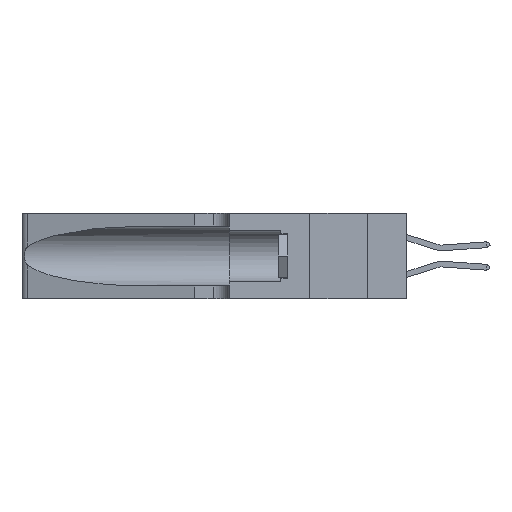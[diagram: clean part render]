
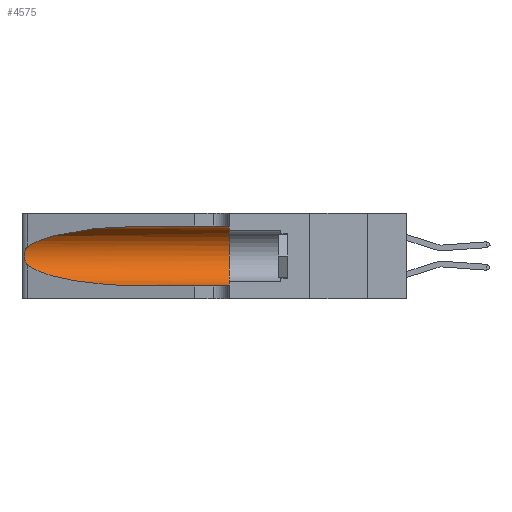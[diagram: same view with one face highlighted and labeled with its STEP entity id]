
A CAD part, left-side view. The second image highlights one B-rep face of the part: STEP entity #4575.
In plain terms, the highlighted cylindrical face has radius 3.308 mm (diameter 6.617 mm), a partial arc.
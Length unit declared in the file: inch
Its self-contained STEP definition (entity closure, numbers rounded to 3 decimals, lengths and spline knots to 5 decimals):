
#116 = CARTESIAN_POINT ( 'NONE',  ( 0.1305, 0.35, 0.05475 ) ) ;
#204 = CARTESIAN_POINT ( 'NONE',  ( 0.25854, 1.2359, 0.20912 ) ) ;
#743 = VERTEX_POINT ( 'NONE', #1763 ) ;
#820 = CARTESIAN_POINT ( 'NONE',  ( 0.1305, 0.35, 0.31525 ) ) ;
#1292 = DIRECTION ( 'NONE',  ( 0., 1., 0. ) ) ;
#1763 = CARTESIAN_POINT ( 'NONE',  ( 0.25487, 1.22718, 0.14631 ) ) ;
#1822 = ORIENTED_EDGE ( 'NONE', *, *, #18909, .T. ) ;
#2095 = EDGE_CURVE ( 'NONE', #21212, #743, #15231, .T. ) ;
#3224 = EDGE_CURVE ( 'NONE', #14481, #21212, #11499, .T. ) ;
#3619 = CARTESIAN_POINT ( 'NONE',  ( 0.1305, 1.61858, 0.05475 ) ) ;
#3789 = CARTESIAN_POINT ( 'NONE',  ( 0.25555, 1.22994, 0.2215 ) ) ;
#3817 = CARTESIAN_POINT ( 'NONE',  ( 0.26018, 1.23835, 0.19895 ) ) ;
#3951 = CARTESIAN_POINT ( 'NONE',  ( 0.25856, 1.23593, 0.16098 ) ) ;
#4509 = CARTESIAN_POINT ( 'NONE',  ( 0.25789, 1.23486, 0.15765 ) ) ;
#4575 = ADVANCED_FACE ( 'NONE', ( #9267 ), #12246, .F. ) ;
#5392 = ORIENTED_EDGE ( 'NONE', *, *, #2095, .T. ) ;
#6337 = ORIENTED_EDGE ( 'NONE', *, *, #8643, .F. ) ;
#6398 = CARTESIAN_POINT ( 'NONE',  ( 0.1305, 0.72297, 0.05475 ) ) ;
#6425 = CARTESIAN_POINT ( 'NONE',  ( 0.25487, 1.22718, 0.22369 ) ) ;
#7022 = VERTEX_POINT ( 'NONE', #20162 ) ;
#7311 = EDGE_CURVE ( 'NONE', #743, #7022, #11792, .T. ) ;
#7464 = CARTESIAN_POINT ( 'NONE',  ( 0.1305, 1.61858, 0.31525 ) ) ;
#7591 = AXIS2_PLACEMENT_3D ( 'NONE', #8154, #1292, #13288 ) ;
#8154 = CARTESIAN_POINT ( 'NONE',  ( 0.1305, 0.35, 0.185 ) ) ;
#8545 = LINE ( 'NONE', #7464, #14473 ) ;
#8599 = EDGE_CURVE ( 'NONE', #14481, #14211, #8545, .T. ) ;
#8643 = EDGE_CURVE ( 'NONE', #14211, #12919, #10958, .T. ) ;
#8984 = CARTESIAN_POINT ( 'NONE',  ( 0.25487, 1.22718, 0.14631 ) ) ;
#9267 = FACE_OUTER_BOUND ( 'NONE', #21830, .T. ) ;
#10089 = CARTESIAN_POINT ( 'NONE',  ( 0.1305, 1.61858, 0.185 ) ) ;
#10958 = CIRCLE ( 'NONE', #7591, 0.13025 ) ;
#11499 =( BOUNDED_CURVE ( )  B_SPLINE_CURVE ( 3, ( #16228, #17680, #14275, #12471 ),
 .UNSPECIFIED., .F., .T. ) 
 B_SPLINE_CURVE_WITH_KNOTS ( ( 4, 4 ),
 ( 1.5708, 2.84003 ),
 .UNSPECIFIED. ) 
 CURVE ( )  GEOMETRIC_REPRESENTATION_ITEM ( )  RATIONAL_B_SPLINE_CURVE ( ( 1., 0.87, 0.87, 1. ) ) 
 REPRESENTATION_ITEM ( '' )  );
#11741 = CARTESIAN_POINT ( 'NONE',  ( 0.18966, 0.96281, 0.05475 ) ) ;
#11792 =( BOUNDED_CURVE ( )  B_SPLINE_CURVE ( 3, ( #8984, #15050, #11741, #6398 ),
 .UNSPECIFIED., .F., .T. ) 
 B_SPLINE_CURVE_WITH_KNOTS ( ( 4, 4 ),
 ( 3.44316, 4.71239 ),
 .UNSPECIFIED. ) 
 CURVE ( )  GEOMETRIC_REPRESENTATION_ITEM ( )  RATIONAL_B_SPLINE_CURVE ( ( 1., 0.87, 0.87, 1. ) ) 
 REPRESENTATION_ITEM ( '' )  );
#12246 = CYLINDRICAL_SURFACE ( 'NONE', #14768, 0.13025 ) ;
#12471 = CARTESIAN_POINT ( 'NONE',  ( 0.25487, 1.22718, 0.22369 ) ) ;
#12919 = VERTEX_POINT ( 'NONE', #116 ) ;
#13288 = DIRECTION ( 'NONE',  ( 0., 0., 1. ) ) ;
#13420 = ORIENTED_EDGE ( 'NONE', *, *, #8599, .F. ) ;
#13934 = CARTESIAN_POINT ( 'NONE',  ( 0.25639, 1.23184, 0.21858 ) ) ;
#14068 = CARTESIAN_POINT ( 'NONE',  ( 0.25787, 1.23484, 0.2124 ) ) ;
#14211 = VERTEX_POINT ( 'NONE', #820 ) ;
#14275 = CARTESIAN_POINT ( 'NONE',  ( 0.2373, 1.15595, 0.28018 ) ) ;
#14473 = VECTOR ( 'NONE', #21308, 39.37008 ) ;
#14481 = VERTEX_POINT ( 'NONE', #17709 ) ;
#14768 = AXIS2_PLACEMENT_3D ( 'NONE', #10089, #16945, #22263 ) ;
#15050 = CARTESIAN_POINT ( 'NONE',  ( 0.2373, 1.15595, 0.08982 ) ) ;
#15213 = CARTESIAN_POINT ( 'NONE',  ( 0.25555, 1.22993, 0.14849 ) ) ;
#15231 = B_SPLINE_CURVE_WITH_KNOTS ( 'NONE', 3,
 ( #15700, #3789, #13934, #14068, #204, #3817, #15857, #17625, #19977, #3951, #4509, #15936, #15213, #16944 ),
 .UNSPECIFIED., .F., .F.,
 ( 4, 2, 2, 2, 2, 2, 4 ),
 ( 0., 0.00027, 0.00053, 0.00107, 0.0016, 0.00187, 0.00214 ),
 .UNSPECIFIED. ) ;
#15674 = ORIENTED_EDGE ( 'NONE', *, *, #7311, .T. ) ;
#15700 = CARTESIAN_POINT ( 'NONE',  ( 0.25487, 1.22718, 0.22369 ) ) ;
#15857 = CARTESIAN_POINT ( 'NONE',  ( 0.26075, 1.23896, 0.19203 ) ) ;
#15867 = VECTOR ( 'NONE', #20923, 39.37008 ) ;
#15936 = CARTESIAN_POINT ( 'NONE',  ( 0.25639, 1.23186, 0.15144 ) ) ;
#16228 = CARTESIAN_POINT ( 'NONE',  ( 0.1305, 0.72297, 0.31525 ) ) ;
#16944 = CARTESIAN_POINT ( 'NONE',  ( 0.25487, 1.22718, 0.14631 ) ) ;
#16945 = DIRECTION ( 'NONE',  ( 0., -1., 0. ) ) ;
#17625 = CARTESIAN_POINT ( 'NONE',  ( 0.26075, 1.23896, 0.178 ) ) ;
#17680 = CARTESIAN_POINT ( 'NONE',  ( 0.18966, 0.96281, 0.31525 ) ) ;
#17709 = CARTESIAN_POINT ( 'NONE',  ( 0.1305, 0.72297, 0.31525 ) ) ;
#18909 = EDGE_CURVE ( 'NONE', #7022, #12919, #20244, .T. ) ;
#19521 = ORIENTED_EDGE ( 'NONE', *, *, #3224, .T. ) ;
#19977 = CARTESIAN_POINT ( 'NONE',  ( 0.26017, 1.23833, 0.17102 ) ) ;
#20162 = CARTESIAN_POINT ( 'NONE',  ( 0.1305, 0.72297, 0.05475 ) ) ;
#20244 = LINE ( 'NONE', #3619, #15867 ) ;
#20923 = DIRECTION ( 'NONE',  ( 0., -1., 0. ) ) ;
#21212 = VERTEX_POINT ( 'NONE', #6425 ) ;
#21308 = DIRECTION ( 'NONE',  ( 0., -1., 0. ) ) ;
#21830 = EDGE_LOOP ( 'NONE', ( #19521, #5392, #15674, #1822, #6337, #13420 ) ) ;
#22263 = DIRECTION ( 'NONE',  ( 0., 0., -1. ) ) ;
